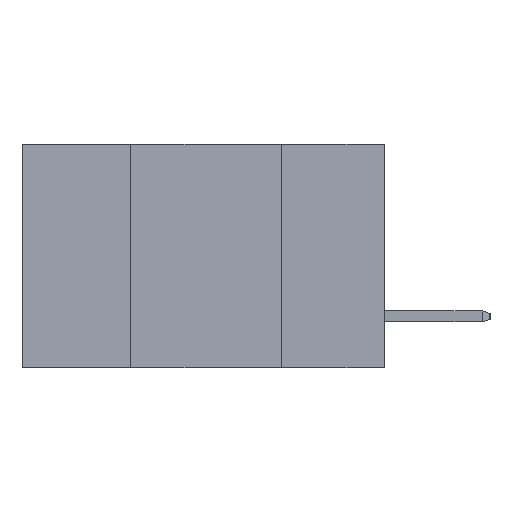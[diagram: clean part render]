
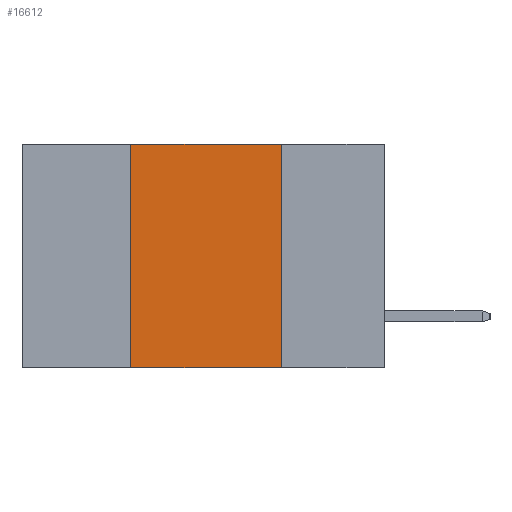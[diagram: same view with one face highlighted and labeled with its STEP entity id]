
A CAD part, left-side view. The second image highlights one B-rep face of the part: STEP entity #16612.
In plain terms, the highlighted planar face has unit normal (-1, 0, 0).
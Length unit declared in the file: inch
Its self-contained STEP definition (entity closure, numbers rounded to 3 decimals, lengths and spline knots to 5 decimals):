
#592 = CARTESIAN_POINT ( 'NONE',  ( 0., 0.17, 0. ) ) ;
#1533 = PLANE ( 'NONE',  #17330 ) ;
#3941 = EDGE_LOOP ( 'NONE', ( #28495, #13817, #7952, #17389 ) ) ;
#4016 = CARTESIAN_POINT ( 'NONE',  ( 0., 0.6, 0. ) ) ;
#5530 = CARTESIAN_POINT ( 'NONE',  ( 0., 0.17, -0.37 ) ) ;
#6018 = DIRECTION ( 'NONE',  ( 0., 0., 1. ) ) ;
#6667 = EDGE_CURVE ( 'NONE', #17591, #12729, #15112, .T. ) ;
#7416 = DIRECTION ( 'NONE',  ( 0., -1., 0. ) ) ;
#7952 = ORIENTED_EDGE ( 'NONE', *, *, #22323, .F. ) ;
#8332 = FACE_OUTER_BOUND ( 'NONE', #3941, .T. ) ;
#8455 = VECTOR ( 'NONE', #14872, 39.37008 ) ;
#9044 = DIRECTION ( 'NONE',  ( 1., 0., 0. ) ) ;
#11048 = CARTESIAN_POINT ( 'NONE',  ( 0., 0.42, 0. ) ) ;
#11229 = CARTESIAN_POINT ( 'NONE',  ( 0., 0.6, -0.37 ) ) ;
#12419 = LINE ( 'NONE', #18509, #19044 ) ;
#12729 = VERTEX_POINT ( 'NONE', #5530 ) ;
#13817 = ORIENTED_EDGE ( 'NONE', *, *, #25393, .F. ) ;
#14563 = LINE ( 'NONE', #17392, #20419 ) ;
#14872 = DIRECTION ( 'NONE',  ( 0., -1., 0. ) ) ;
#15112 = LINE ( 'NONE', #11229, #8455 ) ;
#15455 = VERTEX_POINT ( 'NONE', #24634 ) ;
#15538 = DIRECTION ( 'NONE',  ( 0., 0., -1. ) ) ;
#15675 = EDGE_CURVE ( 'NONE', #15455, #12729, #31192, .T. ) ;
#16612 = ADVANCED_FACE ( 'NONE', ( #8332 ), #1533, .F. ) ;
#17137 = CARTESIAN_POINT ( 'NONE',  ( 0., 0.42, -0.37 ) ) ;
#17330 = AXIS2_PLACEMENT_3D ( 'NONE', #4016, #9044, #26393 ) ;
#17389 = ORIENTED_EDGE ( 'NONE', *, *, #6667, .T. ) ;
#17392 = CARTESIAN_POINT ( 'NONE',  ( 0., 0.6, 0. ) ) ;
#17591 = VERTEX_POINT ( 'NONE', #17137 ) ;
#18509 = CARTESIAN_POINT ( 'NONE',  ( 0., 0.42, 0. ) ) ;
#19044 = VECTOR ( 'NONE', #6018, 39.37008 ) ;
#20419 = VECTOR ( 'NONE', #7416, 39.37008 ) ;
#22323 = EDGE_CURVE ( 'NONE', #17591, #25024, #12419, .T. ) ;
#24634 = CARTESIAN_POINT ( 'NONE',  ( 0., 0.17, 0. ) ) ;
#25024 = VERTEX_POINT ( 'NONE', #11048 ) ;
#25393 = EDGE_CURVE ( 'NONE', #25024, #15455, #14563, .T. ) ;
#25498 = VECTOR ( 'NONE', #15538, 39.37008 ) ;
#26393 = DIRECTION ( 'NONE',  ( 0., 0., -1. ) ) ;
#28495 = ORIENTED_EDGE ( 'NONE', *, *, #15675, .F. ) ;
#31192 = LINE ( 'NONE', #592, #25498 ) ;
